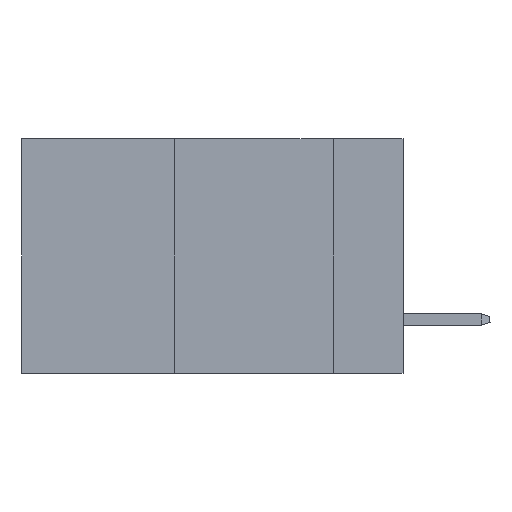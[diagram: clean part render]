
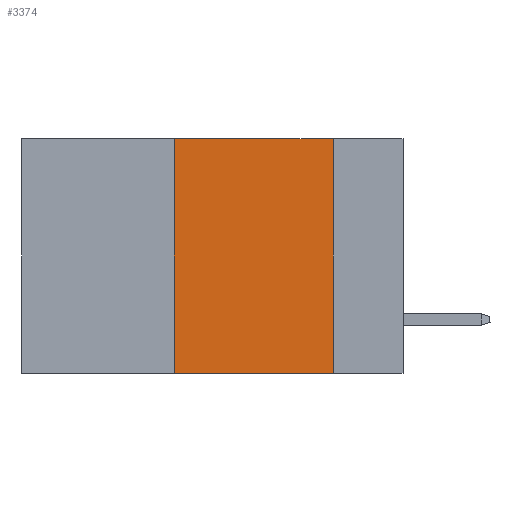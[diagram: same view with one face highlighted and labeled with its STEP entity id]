
A CAD part, left-side view. The second image highlights one B-rep face of the part: STEP entity #3374.
In plain terms, the highlighted planar face has unit normal (-1, 0, 0).
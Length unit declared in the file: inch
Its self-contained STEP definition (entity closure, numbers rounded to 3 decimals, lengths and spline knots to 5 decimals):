
#1577 = CARTESIAN_POINT ( 'NONE',  ( 0., 0.36, 0. ) ) ;
#2698 = CARTESIAN_POINT ( 'NONE',  ( 0., 0.6, 0. ) ) ;
#3074 = DIRECTION ( 'NONE',  ( 0., -1., 0. ) ) ;
#3299 = VERTEX_POINT ( 'NONE', #5237 ) ;
#3374 = ADVANCED_FACE ( 'NONE', ( #14903 ), #5481, .F. ) ;
#3518 = VECTOR ( 'NONE', #9101, 39.37008 ) ;
#3631 = DIRECTION ( 'NONE',  ( 0., 0., -1. ) ) ;
#4297 = LINE ( 'NONE', #11868, #22562 ) ;
#5237 = CARTESIAN_POINT ( 'NONE',  ( 0., 0.11, -0.37 ) ) ;
#5481 = PLANE ( 'NONE',  #24229 ) ;
#5830 = CARTESIAN_POINT ( 'NONE',  ( 0., 0.11, 0. ) ) ;
#6614 = ORIENTED_EDGE ( 'NONE', *, *, #18790, .F. ) ;
#7350 = DIRECTION ( 'NONE',  ( 0., -1., 0. ) ) ;
#8744 = LINE ( 'NONE', #18490, #3518 ) ;
#9040 = ORIENTED_EDGE ( 'NONE', *, *, #13339, .T. ) ;
#9101 = DIRECTION ( 'NONE',  ( 0., 0., -1. ) ) ;
#9208 = CARTESIAN_POINT ( 'NONE',  ( 0., 0.6, -0.37 ) ) ;
#9282 = VECTOR ( 'NONE', #3074, 39.37008 ) ;
#11195 = LINE ( 'NONE', #9208, #22036 ) ;
#11617 = ORIENTED_EDGE ( 'NONE', *, *, #23747, .F. ) ;
#11868 = CARTESIAN_POINT ( 'NONE',  ( 0., 0.36, 0. ) ) ;
#13055 = CARTESIAN_POINT ( 'NONE',  ( 0., 0.6, 0. ) ) ;
#13339 = EDGE_CURVE ( 'NONE', #15939, #3299, #11195, .T. ) ;
#14272 = EDGE_CURVE ( 'NONE', #15289, #3299, #8744, .T. ) ;
#14903 = FACE_OUTER_BOUND ( 'NONE', #17833, .T. ) ;
#15200 = ORIENTED_EDGE ( 'NONE', *, *, #14272, .F. ) ;
#15289 = VERTEX_POINT ( 'NONE', #5830 ) ;
#15441 = CARTESIAN_POINT ( 'NONE',  ( 0., 0.36, -0.37 ) ) ;
#15811 = DIRECTION ( 'NONE',  ( 0., 0., 1. ) ) ;
#15939 = VERTEX_POINT ( 'NONE', #15441 ) ;
#17433 = VERTEX_POINT ( 'NONE', #1577 ) ;
#17833 = EDGE_LOOP ( 'NONE', ( #15200, #11617, #6614, #9040 ) ) ;
#18490 = CARTESIAN_POINT ( 'NONE',  ( 0., 0.11, 0. ) ) ;
#18790 = EDGE_CURVE ( 'NONE', #15939, #17433, #4297, .T. ) ;
#20554 = DIRECTION ( 'NONE',  ( 1., 0., 0. ) ) ;
#21712 = LINE ( 'NONE', #2698, #9282 ) ;
#22036 = VECTOR ( 'NONE', #7350, 39.37008 ) ;
#22562 = VECTOR ( 'NONE', #15811, 39.37008 ) ;
#23747 = EDGE_CURVE ( 'NONE', #17433, #15289, #21712, .T. ) ;
#24229 = AXIS2_PLACEMENT_3D ( 'NONE', #13055, #20554, #3631 ) ;
